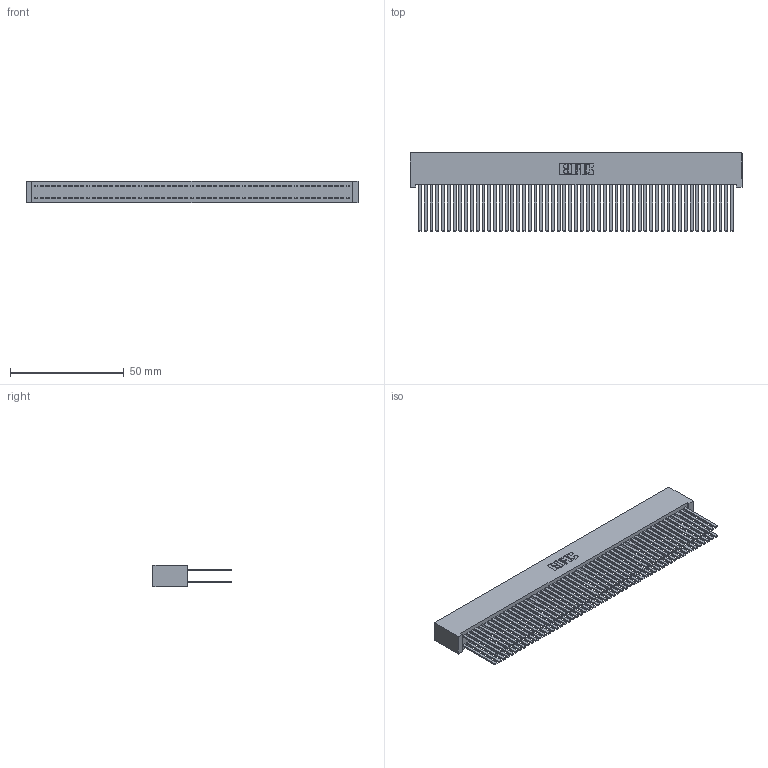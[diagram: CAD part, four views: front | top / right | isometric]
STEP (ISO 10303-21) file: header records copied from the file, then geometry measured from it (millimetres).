
FILE_DESCRIPTION (( 'STEP AP203' ), '1' );
FILE_NAME ('392-110-544-201.STEP', '2018-08-18T21:51:00', ( '' ), ( '' ), 'SwSTEP 2.0', 'SolidWorks 2016', '' );
FILE_SCHEMA (( 'CONFIG_CONTROL_DESIGN' ));
Length unit declared in the file: inch
Products named in the file (3): 342 Part_Lugless; 345-292-001_345-293-144; 392-110-544-201
Assembly tree (111 placements, depth 2):
  392-110-544-201
    342 Part_Lugless
    345-292-001_345-293-144  x110
Bounding box: 145.95 x 34.3 x 9.4 mm (x, y, z)
Volume: 15156.5 mm3; surface area: 29707.9 mm2
Topology: 111 solids, 111 shells, 5162 faces, 15345 edges, 10082 vertices
Faces by surface type: plane 3582, cylinder 1580
Entity records: 33109 total; most frequent: CARTESIAN_POINT 5466, ORIENTED_EDGE 5402, DIRECTION 4637, EDGE_CURVE 2701, LINE 2585, VECTOR 2585, VERTEX_POINT 1798, AXIS2_PLACEMENT_3D 1026
